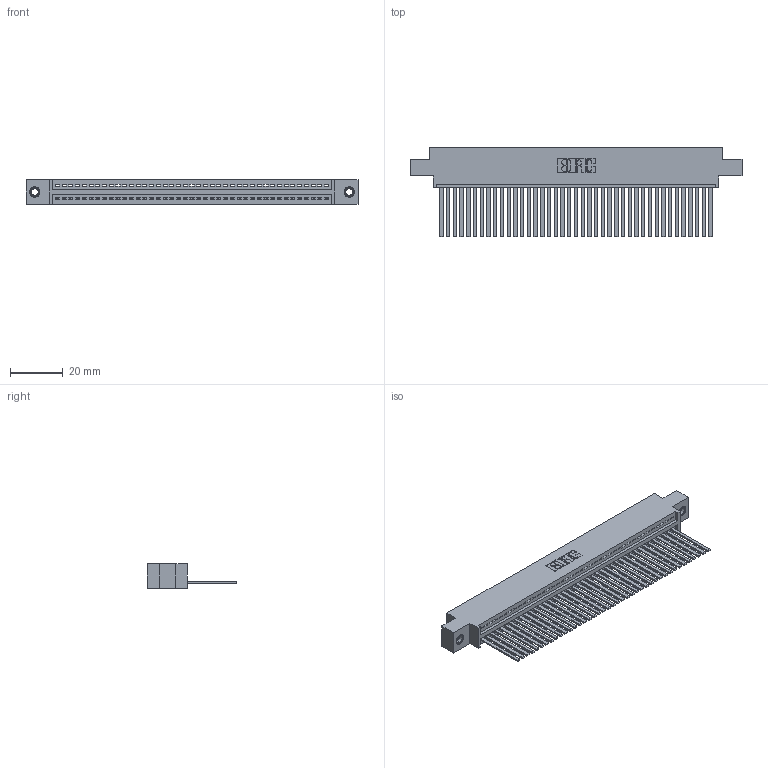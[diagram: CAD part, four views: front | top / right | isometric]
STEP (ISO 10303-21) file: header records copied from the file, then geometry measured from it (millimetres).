
FILE_DESCRIPTION (( 'STEP AP203' ), '1' );
FILE_NAME ('345-041-544-607.STEP', '2018-09-05T09:13:04', ( '' ), ( '' ), 'SwSTEP 2.0', 'SolidWorks 2016', '' );
FILE_SCHEMA (( 'CONFIG_CONTROL_DESIGN' ));
Length unit declared in the file: inch
Products named in the file (4): 345 Part_0.170 Offset - 0.156 Dia-TI; 345-292-001_345-293-144; 345-250-001_345-250-005-103; 345-041-544-607
Assembly tree (44 placements, depth 2):
  345-041-544-607
    345 Part_0.170 Offset - 0.156 Dia-TI
    345-292-001_345-293-144  x41
    345-250-001_345-250-005-103  x2
Bounding box: 125.35 x 33.96 x 9.4 mm (x, y, z)
Volume: 12245.5 mm3; surface area: 17844.2 mm2
Topology: 44 solids, 44 shells, 2322 faces, 6967 edges, 4582 vertices
Faces by surface type: plane 1592, cylinder 714, cone 12, torus 4
Entity records: 32126 total; most frequent: CARTESIAN_POINT 5546, ORIENTED_EDGE 5514, DIRECTION 4869, EDGE_CURVE 2757, VECTOR 2445, LINE 2445, VERTEX_POINT 1832, AXIS2_PLACEMENT_3D 1212
